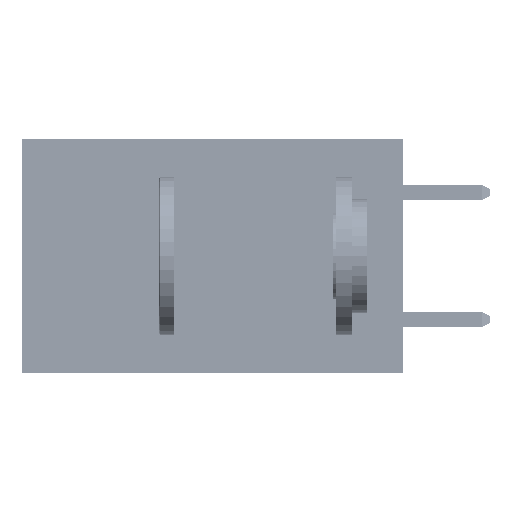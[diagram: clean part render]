
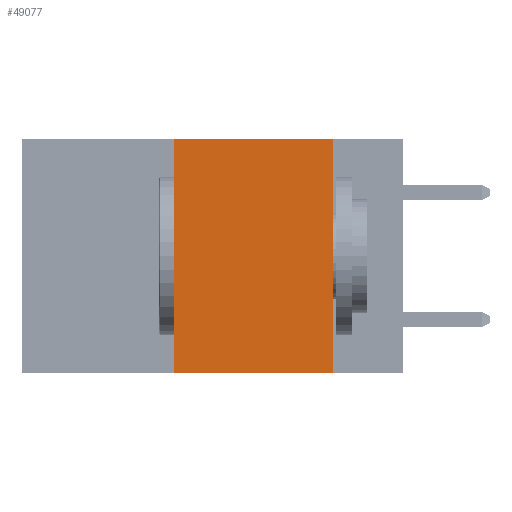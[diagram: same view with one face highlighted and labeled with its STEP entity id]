
A CAD part, left-side view. The second image highlights one B-rep face of the part: STEP entity #49077.
In plain terms, the highlighted planar face has unit normal (-1, 0, 0).
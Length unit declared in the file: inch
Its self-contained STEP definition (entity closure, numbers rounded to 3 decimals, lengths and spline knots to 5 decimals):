
#679 = CARTESIAN_POINT ( 'NONE',  ( 0., 0.6, 0. ) ) ;
#4474 = PLANE ( 'NONE',  #28845 ) ;
#5317 = CARTESIAN_POINT ( 'NONE',  ( 0., 0.11, 0. ) ) ;
#6065 = CARTESIAN_POINT ( 'NONE',  ( 0., 0.36, 0. ) ) ;
#7423 = DIRECTION ( 'NONE',  ( 0., -1., 0. ) ) ;
#7434 = VERTEX_POINT ( 'NONE', #14787 ) ;
#8420 = EDGE_CURVE ( 'NONE', #33176, #7434, #50952, .T. ) ;
#10295 = EDGE_CURVE ( 'NONE', #7434, #46216, #38939, .T. ) ;
#10937 = VERTEX_POINT ( 'NONE', #43527 ) ;
#11608 = LINE ( 'NONE', #32458, #46972 ) ;
#12787 = ORIENTED_EDGE ( 'NONE', *, *, #8420, .F. ) ;
#14787 = CARTESIAN_POINT ( 'NONE',  ( 0., 0.36, 0. ) ) ;
#14896 = LINE ( 'NONE', #16303, #32237 ) ;
#15302 = CARTESIAN_POINT ( 'NONE',  ( 0., 0.36, -0.37 ) ) ;
#16303 = CARTESIAN_POINT ( 'NONE',  ( 0., 0.11, 0. ) ) ;
#26268 = DIRECTION ( 'NONE',  ( 0., 0., 1. ) ) ;
#28845 = AXIS2_PLACEMENT_3D ( 'NONE', #679, #39992, #32152 ) ;
#32075 = DIRECTION ( 'NONE',  ( 0., 0., -1. ) ) ;
#32152 = DIRECTION ( 'NONE',  ( 0., 0., -1. ) ) ;
#32237 = VECTOR ( 'NONE', #32075, 39.37008 ) ;
#32458 = CARTESIAN_POINT ( 'NONE',  ( 0., 0.6, -0.37 ) ) ;
#32731 = VECTOR ( 'NONE', #7423, 39.37008 ) ;
#33176 = VERTEX_POINT ( 'NONE', #15302 ) ;
#34856 = EDGE_CURVE ( 'NONE', #33176, #10937, #11608, .T. ) ;
#35604 = CARTESIAN_POINT ( 'NONE',  ( 0., 0.6, 0. ) ) ;
#37246 = VECTOR ( 'NONE', #26268, 39.37008 ) ;
#38939 = LINE ( 'NONE', #35604, #32731 ) ;
#39992 = DIRECTION ( 'NONE',  ( 1., 0., 0. ) ) ;
#40006 = FACE_OUTER_BOUND ( 'NONE', #50104, .T. ) ;
#40494 = EDGE_CURVE ( 'NONE', #46216, #10937, #14896, .T. ) ;
#41904 = ORIENTED_EDGE ( 'NONE', *, *, #10295, .F. ) ;
#42142 = ORIENTED_EDGE ( 'NONE', *, *, #34856, .T. ) ;
#43527 = CARTESIAN_POINT ( 'NONE',  ( 0., 0.11, -0.37 ) ) ;
#43786 = DIRECTION ( 'NONE',  ( 0., -1., 0. ) ) ;
#46216 = VERTEX_POINT ( 'NONE', #5317 ) ;
#46972 = VECTOR ( 'NONE', #43786, 39.37008 ) ;
#48810 = ORIENTED_EDGE ( 'NONE', *, *, #40494, .F. ) ;
#49077 = ADVANCED_FACE ( 'NONE', ( #40006 ), #4474, .F. ) ;
#50104 = EDGE_LOOP ( 'NONE', ( #48810, #41904, #12787, #42142 ) ) ;
#50952 = LINE ( 'NONE', #6065, #37246 ) ;
